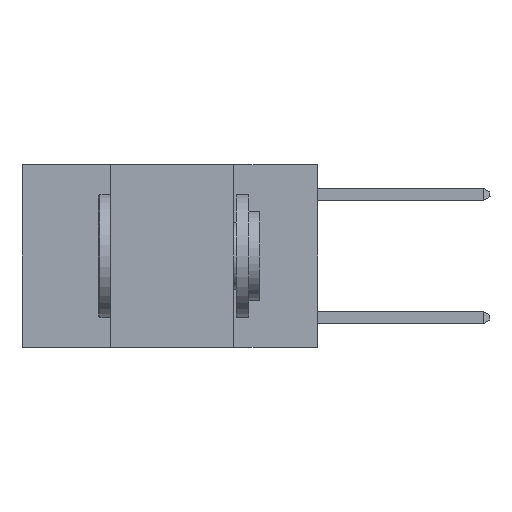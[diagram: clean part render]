
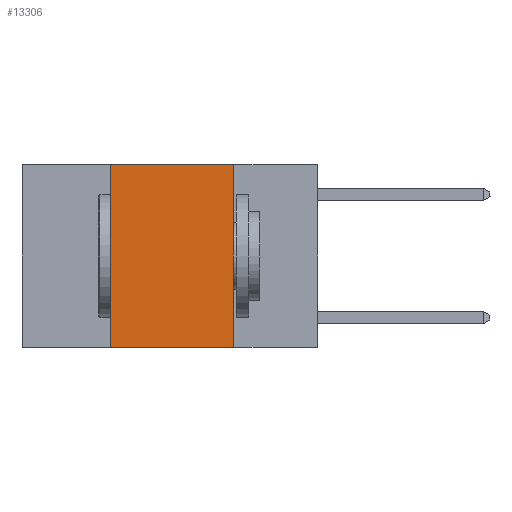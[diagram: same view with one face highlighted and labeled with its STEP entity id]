
A CAD part, left-side view. The second image highlights one B-rep face of the part: STEP entity #13306.
In plain terms, the highlighted planar face has unit normal (-1, 0, 0).
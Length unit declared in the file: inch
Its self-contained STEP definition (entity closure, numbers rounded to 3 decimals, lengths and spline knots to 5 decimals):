
#101 = FACE_OUTER_BOUND ( 'NONE', #10069, .T. ) ;
#250 = VECTOR ( 'NONE', #18444, 39.37008 ) ;
#1788 = ORIENTED_EDGE ( 'NONE', *, *, #3900, .F. ) ;
#1994 = CARTESIAN_POINT ( 'NONE',  ( 0., 0.6, 0. ) ) ;
#2484 = EDGE_CURVE ( 'NONE', #13475, #11283, #3962, .T. ) ;
#3900 = EDGE_CURVE ( 'NONE', #23428, #13475, #19416, .T. ) ;
#3962 = LINE ( 'NONE', #16661, #250 ) ;
#5548 = DIRECTION ( 'NONE',  ( 0., 0., 1. ) ) ;
#5610 = LINE ( 'NONE', #17739, #16155 ) ;
#6593 = CARTESIAN_POINT ( 'NONE',  ( 0., 0.6, 0. ) ) ;
#7324 = CARTESIAN_POINT ( 'NONE',  ( 0., 0.42, 0. ) ) ;
#9135 = VECTOR ( 'NONE', #5548, 39.37008 ) ;
#9257 = DIRECTION ( 'NONE',  ( 1., 0., 0. ) ) ;
#9568 = VECTOR ( 'NONE', #11832, 39.37008 ) ;
#10069 = EDGE_LOOP ( 'NONE', ( #14490, #1788, #15746, #14433 ) ) ;
#11283 = VERTEX_POINT ( 'NONE', #15462 ) ;
#11832 = DIRECTION ( 'NONE',  ( 0., -1., 0. ) ) ;
#12688 = PLANE ( 'NONE',  #13750 ) ;
#13306 = ADVANCED_FACE ( 'NONE', ( #101 ), #12688, .F. ) ;
#13475 = VERTEX_POINT ( 'NONE', #18956 ) ;
#13750 = AXIS2_PLACEMENT_3D ( 'NONE', #1994, #9257, #16497 ) ;
#14433 = ORIENTED_EDGE ( 'NONE', *, *, #16734, .T. ) ;
#14490 = ORIENTED_EDGE ( 'NONE', *, *, #2484, .F. ) ;
#15462 = CARTESIAN_POINT ( 'NONE',  ( 0., 0.17, -0.37 ) ) ;
#15490 = CARTESIAN_POINT ( 'NONE',  ( 0., 0.42, -0.37 ) ) ;
#15746 = ORIENTED_EDGE ( 'NONE', *, *, #21076, .F. ) ;
#16155 = VECTOR ( 'NONE', #23339, 39.37008 ) ;
#16228 = LINE ( 'NONE', #7324, #9135 ) ;
#16497 = DIRECTION ( 'NONE',  ( 0., 0., -1. ) ) ;
#16661 = CARTESIAN_POINT ( 'NONE',  ( 0., 0.17, 0. ) ) ;
#16734 = EDGE_CURVE ( 'NONE', #17982, #11283, #5610, .T. ) ;
#17739 = CARTESIAN_POINT ( 'NONE',  ( 0., 0.6, -0.37 ) ) ;
#17755 = CARTESIAN_POINT ( 'NONE',  ( 0., 0.42, 0. ) ) ;
#17982 = VERTEX_POINT ( 'NONE', #15490 ) ;
#18444 = DIRECTION ( 'NONE',  ( 0., 0., -1. ) ) ;
#18956 = CARTESIAN_POINT ( 'NONE',  ( 0., 0.17, 0. ) ) ;
#19416 = LINE ( 'NONE', #6593, #9568 ) ;
#21076 = EDGE_CURVE ( 'NONE', #17982, #23428, #16228, .T. ) ;
#23339 = DIRECTION ( 'NONE',  ( 0., -1., 0. ) ) ;
#23428 = VERTEX_POINT ( 'NONE', #17755 ) ;
